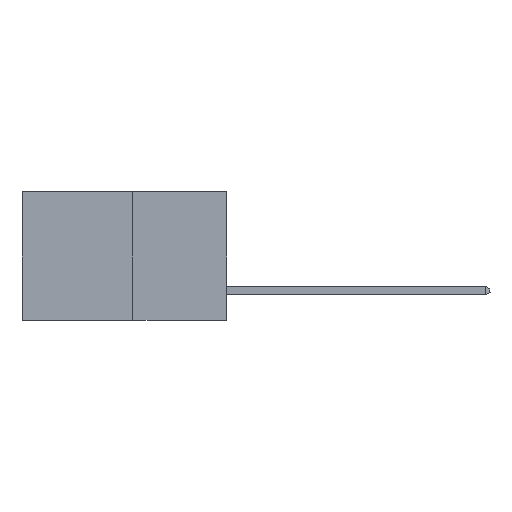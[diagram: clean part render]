
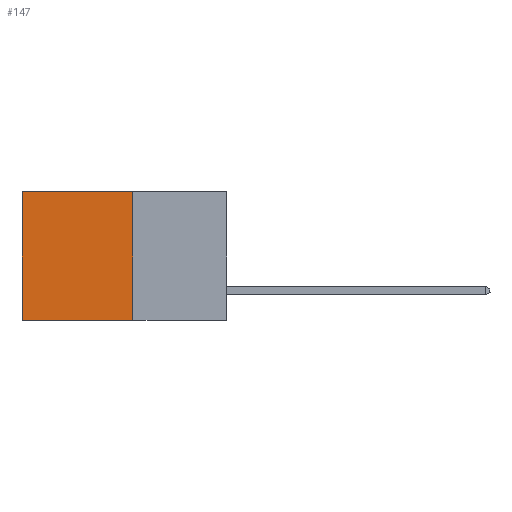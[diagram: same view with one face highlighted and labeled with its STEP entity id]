
A CAD part, left-side view. The second image highlights one B-rep face of the part: STEP entity #147.
In plain terms, the highlighted planar face has unit normal (-1, 0, 0).
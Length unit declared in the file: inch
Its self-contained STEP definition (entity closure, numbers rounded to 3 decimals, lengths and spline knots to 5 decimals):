
#2 = VERTEX_POINT ( 'NONE', #5313 ) ;
#147 = ADVANCED_FACE ( 'NONE', ( #2631 ), #9144, .F. ) ;
#157 = VECTOR ( 'NONE', #9965, 39.37008 ) ;
#440 = CARTESIAN_POINT ( 'NONE',  ( 0.277, 0.59, -0.37 ) ) ;
#1164 = DIRECTION ( 'NONE',  ( 0., 0., -1. ) ) ;
#1308 = ORIENTED_EDGE ( 'NONE', *, *, #3278, .T. ) ;
#1514 = CARTESIAN_POINT ( 'NONE',  ( 0.277, 0.27, -0.37 ) ) ;
#2030 = CARTESIAN_POINT ( 'NONE',  ( 0.277, 0.27, 0. ) ) ;
#2588 = VECTOR ( 'NONE', #3489, 39.37008 ) ;
#2631 = FACE_OUTER_BOUND ( 'NONE', #5548, .T. ) ;
#3278 = EDGE_CURVE ( 'NONE', #4599, #11890, #6392, .T. ) ;
#3489 = DIRECTION ( 'NONE',  ( 0., 1., 0. ) ) ;
#4378 = EDGE_CURVE ( 'NONE', #6387, #2, #9935, .T. ) ;
#4416 = CARTESIAN_POINT ( 'NONE',  ( 0.277, 0.27, -0.37 ) ) ;
#4599 = VERTEX_POINT ( 'NONE', #2030 ) ;
#4904 = EDGE_CURVE ( 'NONE', #11890, #2, #5653, .T. ) ;
#4913 = DIRECTION ( 'NONE',  ( 0., 0., -1. ) ) ;
#5313 = CARTESIAN_POINT ( 'NONE',  ( 0.277, 0.59, -0.37 ) ) ;
#5548 = EDGE_LOOP ( 'NONE', ( #6700, #9148, #11270, #1308 ) ) ;
#5653 = LINE ( 'NONE', #440, #157 ) ;
#5884 = CARTESIAN_POINT ( 'NONE',  ( 0.277, 0.27, -0.37 ) ) ;
#6387 = VERTEX_POINT ( 'NONE', #11024 ) ;
#6392 = LINE ( 'NONE', #11395, #10748 ) ;
#6700 = ORIENTED_EDGE ( 'NONE', *, *, #4904, .T. ) ;
#8079 = CARTESIAN_POINT ( 'NONE',  ( 0.277, 0.59, 0. ) ) ;
#8691 = AXIS2_PLACEMENT_3D ( 'NONE', #1514, #11014, #1164 ) ;
#8947 = VECTOR ( 'NONE', #4913, 39.37008 ) ;
#9144 = PLANE ( 'NONE',  #8691 ) ;
#9148 = ORIENTED_EDGE ( 'NONE', *, *, #4378, .F. ) ;
#9935 = LINE ( 'NONE', #4416, #2588 ) ;
#9965 = DIRECTION ( 'NONE',  ( 0., 0., -1. ) ) ;
#10538 = DIRECTION ( 'NONE',  ( 0., 1., 0. ) ) ;
#10748 = VECTOR ( 'NONE', #10538, 39.37008 ) ;
#11014 = DIRECTION ( 'NONE',  ( 1., 0., 0. ) ) ;
#11024 = CARTESIAN_POINT ( 'NONE',  ( 0.277, 0.27, -0.37 ) ) ;
#11270 = ORIENTED_EDGE ( 'NONE', *, *, #12381, .F. ) ;
#11321 = LINE ( 'NONE', #5884, #8947 ) ;
#11395 = CARTESIAN_POINT ( 'NONE',  ( 0.277, 0.27, 0. ) ) ;
#11890 = VERTEX_POINT ( 'NONE', #8079 ) ;
#12381 = EDGE_CURVE ( 'NONE', #4599, #6387, #11321, .T. ) ;
